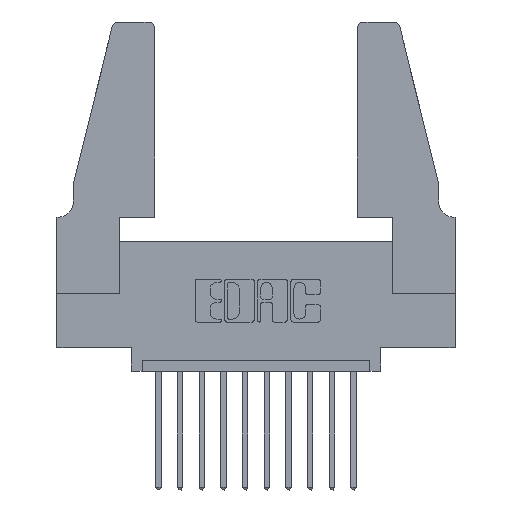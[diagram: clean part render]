
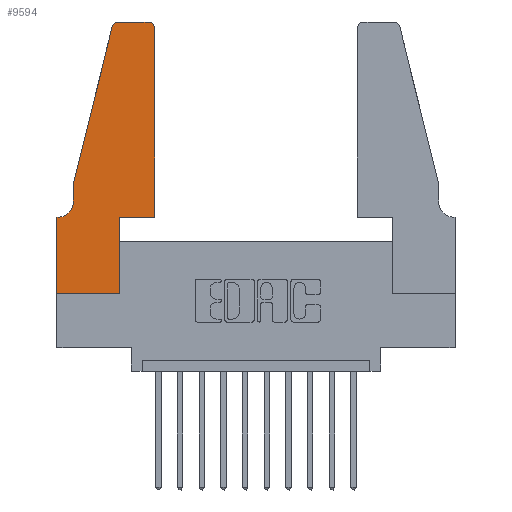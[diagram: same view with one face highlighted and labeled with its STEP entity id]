
A CAD part, top view. The second image highlights one B-rep face of the part: STEP entity #9594.
In plain terms, the highlighted planar face has unit normal (0, 0, 1).
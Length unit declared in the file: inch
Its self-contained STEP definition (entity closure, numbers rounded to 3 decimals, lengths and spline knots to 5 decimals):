
#163 = CARTESIAN_POINT ( 'NONE',  ( 0.0055, 0.42, 0.37 ) ) ;
#267 = VECTOR ( 'NONE', #6764, 39.37008 ) ;
#630 = VECTOR ( 'NONE', #2230, 39.37008 ) ;
#653 = ORIENTED_EDGE ( 'NONE', *, *, #1387, .T. ) ;
#659 = DIRECTION ( 'NONE',  ( 0., -1., 0. ) ) ;
#1100 = VECTOR ( 'NONE', #659, 39.37008 ) ;
#1162 = VERTEX_POINT ( 'NONE', #11786 ) ;
#1344 = CARTESIAN_POINT ( 'NONE',  ( 0., 0., 0.37 ) ) ;
#1387 = EDGE_CURVE ( 'NONE', #10975, #7943, #9159, .T. ) ;
#1494 = CARTESIAN_POINT ( 'NONE',  ( 0.0755, 0.35, 0.37 ) ) ;
#1805 = VERTEX_POINT ( 'NONE', #11975 ) ;
#1954 = EDGE_CURVE ( 'NONE', #1805, #3386, #11535, .T. ) ;
#2007 = DIRECTION ( 'NONE',  ( 0., 1., 0. ) ) ;
#2018 = LINE ( 'NONE', #10842, #630 ) ;
#2030 = ORIENTED_EDGE ( 'NONE', *, *, #6044, .T. ) ;
#2110 = VECTOR ( 'NONE', #6640, 39.37008 ) ;
#2230 = DIRECTION ( 'NONE',  ( 0., 1., 0. ) ) ;
#2524 = DIRECTION ( 'NONE',  ( 1., 0., 0. ) ) ;
#2702 = LINE ( 'NONE', #6024, #11753 ) ;
#2727 = DIRECTION ( 'NONE',  ( 1., 0., 0. ) ) ;
#2738 = AXIS2_PLACEMENT_3D ( 'NONE', #11892, #10449, #4081 ) ;
#2814 = DIRECTION ( 'NONE',  ( -1., 0., 0. ) ) ;
#2839 = ORIENTED_EDGE ( 'NONE', *, *, #5790, .T. ) ;
#2948 = CARTESIAN_POINT ( 'NONE',  ( 0.2865, 0., 0.37 ) ) ;
#2955 = ORIENTED_EDGE ( 'NONE', *, *, #10158, .T. ) ;
#3348 = CARTESIAN_POINT ( 'NONE',  ( 0.0755, 0.5, 0.37 ) ) ;
#3362 = EDGE_CURVE ( 'NONE', #1162, #7423, #5881, .T. ) ;
#3386 = VERTEX_POINT ( 'NONE', #11597 ) ;
#3609 = ORIENTED_EDGE ( 'NONE', *, *, #1954, .T. ) ;
#3817 = EDGE_CURVE ( 'NONE', #12356, #6708, #12935, .T. ) ;
#3822 = AXIS2_PLACEMENT_3D ( 'NONE', #7949, #10063, #13263 ) ;
#3924 = EDGE_CURVE ( 'NONE', #11133, #7813, #2702, .T. ) ;
#4047 = FACE_OUTER_BOUND ( 'NONE', #14105, .T. ) ;
#4081 = DIRECTION ( 'NONE',  ( 1., 0., 0. ) ) ;
#4278 = CARTESIAN_POINT ( 'NONE',  ( 0.0055, 0.35, 0.37 ) ) ;
#4498 = DIRECTION ( 'NONE',  ( 0., 0., -1. ) ) ;
#4851 = CARTESIAN_POINT ( 'NONE',  ( 0.4205, 1.22, 0.37 ) ) ;
#5460 = CARTESIAN_POINT ( 'NONE',  ( 0.4505, 0.35, 0.37 ) ) ;
#5586 = EDGE_CURVE ( 'NONE', #3386, #10975, #9803, .T. ) ;
#5712 = DIRECTION ( 'NONE',  ( -1., 0., 0. ) ) ;
#5790 = EDGE_CURVE ( 'NONE', #6708, #12091, #10637, .T. ) ;
#5863 = LINE ( 'NONE', #1494, #9423 ) ;
#5881 = LINE ( 'NONE', #9415, #9441 ) ;
#6024 = CARTESIAN_POINT ( 'NONE',  ( 0., 0., 0.37 ) ) ;
#6044 = EDGE_CURVE ( 'NONE', #7813, #13480, #11342, .T. ) ;
#6135 = EDGE_CURVE ( 'NONE', #12091, #1162, #6866, .T. ) ;
#6640 = DIRECTION ( 'NONE',  ( 1., 0., 0. ) ) ;
#6708 = VERTEX_POINT ( 'NONE', #5460 ) ;
#6764 = DIRECTION ( 'NONE',  ( -0.239, -0.971, 0. ) ) ;
#6866 = CIRCLE ( 'NONE', #11970, 0.03 ) ;
#7185 = ORIENTED_EDGE ( 'NONE', *, *, #6135, .T. ) ;
#7298 = ORIENTED_EDGE ( 'NONE', *, *, #8609, .T. ) ;
#7365 = CARTESIAN_POINT ( 'NONE',  ( 0.4505, 0.35, 0.37 ) ) ;
#7423 = VERTEX_POINT ( 'NONE', #8894 ) ;
#7748 = VECTOR ( 'NONE', #2007, 39.37008 ) ;
#7813 = VERTEX_POINT ( 'NONE', #1344 ) ;
#7849 = PLANE ( 'NONE',  #3822 ) ;
#7943 = VERTEX_POINT ( 'NONE', #4278 ) ;
#7949 = CARTESIAN_POINT ( 'NONE',  ( 0., 0.35, 0.37 ) ) ;
#8072 = DIRECTION ( 'NONE',  ( 0., -1., 0. ) ) ;
#8389 = ORIENTED_EDGE ( 'NONE', *, *, #12472, .T. ) ;
#8500 = ORIENTED_EDGE ( 'NONE', *, *, #3362, .T. ) ;
#8609 = EDGE_CURVE ( 'NONE', #7423, #1805, #9896, .T. ) ;
#8650 = ORIENTED_EDGE ( 'NONE', *, *, #3924, .T. ) ;
#8894 = CARTESIAN_POINT ( 'NONE',  ( 0.284, 1.25, 0.37 ) ) ;
#9159 = CIRCLE ( 'NONE', #12444, 0.07 ) ;
#9218 = ORIENTED_EDGE ( 'NONE', *, *, #3817, .T. ) ;
#9415 = CARTESIAN_POINT ( 'NONE',  ( 0.2605, 1.25, 0.37 ) ) ;
#9423 = VECTOR ( 'NONE', #13587, 39.37008 ) ;
#9441 = VECTOR ( 'NONE', #2814, 39.37008 ) ;
#9594 = ADVANCED_FACE ( 'NONE', ( #4047 ), #7849, .T. ) ;
#9803 = LINE ( 'NONE', #13655, #1100 ) ;
#9835 = CARTESIAN_POINT ( 'NONE',  ( 0.4505, 1.22, 0.37 ) ) ;
#9896 = CIRCLE ( 'NONE', #2738, 0.03 ) ;
#10018 = CARTESIAN_POINT ( 'NONE',  ( 0.2865, 0.35, 0.37 ) ) ;
#10063 = DIRECTION ( 'NONE',  ( 0., 0., 1. ) ) ;
#10158 = EDGE_CURVE ( 'NONE', #13480, #12356, #2018, .T. ) ;
#10449 = DIRECTION ( 'NONE',  ( 0., 0., 1. ) ) ;
#10637 = LINE ( 'NONE', #7365, #7748 ) ;
#10842 = CARTESIAN_POINT ( 'NONE',  ( 0.2865, 0.35, 0.37 ) ) ;
#10975 = VERTEX_POINT ( 'NONE', #14089 ) ;
#11133 = VERTEX_POINT ( 'NONE', #11279 ) ;
#11205 = CARTESIAN_POINT ( 'NONE',  ( 0.4505, 0.35, 0.37 ) ) ;
#11279 = CARTESIAN_POINT ( 'NONE',  ( 0., 0.35, 0.37 ) ) ;
#11342 = LINE ( 'NONE', #13217, #2110 ) ;
#11535 = LINE ( 'NONE', #3348, #267 ) ;
#11597 = CARTESIAN_POINT ( 'NONE',  ( 0.0755, 0.5, 0.37 ) ) ;
#11753 = VECTOR ( 'NONE', #8072, 39.37008 ) ;
#11786 = CARTESIAN_POINT ( 'NONE',  ( 0.4205, 1.25, 0.37 ) ) ;
#11892 = CARTESIAN_POINT ( 'NONE',  ( 0.284, 1.22, 0.37 ) ) ;
#11923 = VECTOR ( 'NONE', #2524, 39.37008 ) ;
#11970 = AXIS2_PLACEMENT_3D ( 'NONE', #4851, #12403, #2727 ) ;
#11975 = CARTESIAN_POINT ( 'NONE',  ( 0.25487, 1.22718, 0.37 ) ) ;
#12091 = VERTEX_POINT ( 'NONE', #9835 ) ;
#12356 = VERTEX_POINT ( 'NONE', #10018 ) ;
#12403 = DIRECTION ( 'NONE',  ( 0., 0., 1. ) ) ;
#12444 = AXIS2_PLACEMENT_3D ( 'NONE', #163, #4498, #5712 ) ;
#12472 = EDGE_CURVE ( 'NONE', #7943, #11133, #5863, .T. ) ;
#12774 = ORIENTED_EDGE ( 'NONE', *, *, #5586, .T. ) ;
#12935 = LINE ( 'NONE', #11205, #11923 ) ;
#13217 = CARTESIAN_POINT ( 'NONE',  ( 0., 0., 0.37 ) ) ;
#13263 = DIRECTION ( 'NONE',  ( 1., 0., 0. ) ) ;
#13480 = VERTEX_POINT ( 'NONE', #2948 ) ;
#13587 = DIRECTION ( 'NONE',  ( -1., 0., 0. ) ) ;
#13655 = CARTESIAN_POINT ( 'NONE',  ( 0.0755, 0.5, 0.37 ) ) ;
#14089 = CARTESIAN_POINT ( 'NONE',  ( 0.0755, 0.42, 0.37 ) ) ;
#14105 = EDGE_LOOP ( 'NONE', ( #8500, #7298, #3609, #12774, #653, #8389, #8650, #2030, #2955, #9218, #2839, #7185 ) ) ;
